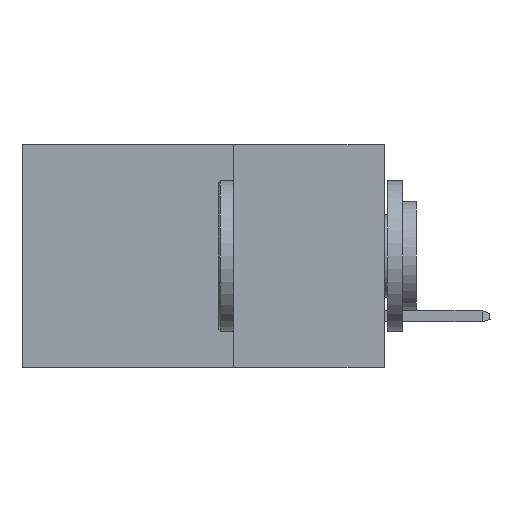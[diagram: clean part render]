
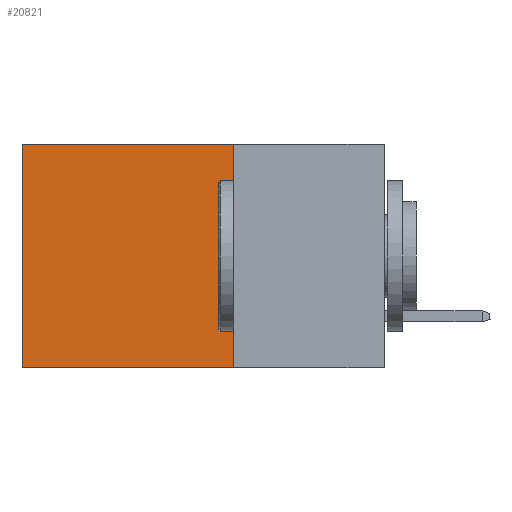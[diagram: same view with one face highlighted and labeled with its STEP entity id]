
A CAD part, left-side view. The second image highlights one B-rep face of the part: STEP entity #20821.
In plain terms, the highlighted planar face has unit normal (-1, 0, 0).
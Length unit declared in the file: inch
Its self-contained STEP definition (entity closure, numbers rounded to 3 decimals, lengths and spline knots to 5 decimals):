
#417 = VECTOR ( 'NONE', #20876, 39.37008 ) ;
#2140 = ORIENTED_EDGE ( 'NONE', *, *, #23260, .T. ) ;
#3273 = CARTESIAN_POINT ( 'NONE',  ( 0.298, 0.25, -0.37 ) ) ;
#4256 = EDGE_LOOP ( 'NONE', ( #18175, #8787, #15003, #2140 ) ) ;
#5755 = VERTEX_POINT ( 'NONE', #19943 ) ;
#6145 = CARTESIAN_POINT ( 'NONE',  ( 0.298, 0.25, 0. ) ) ;
#6293 = DIRECTION ( 'NONE',  ( 0., 0., -1. ) ) ;
#7653 = EDGE_CURVE ( 'NONE', #23555, #8686, #29731, .T. ) ;
#8686 = VERTEX_POINT ( 'NONE', #3273 ) ;
#8787 = ORIENTED_EDGE ( 'NONE', *, *, #19134, .F. ) ;
#10537 = CARTESIAN_POINT ( 'NONE',  ( 0.298, 0.25, 0. ) ) ;
#11476 = DIRECTION ( 'NONE',  ( 0., 0., -1. ) ) ;
#13625 = LINE ( 'NONE', #18662, #417 ) ;
#13712 = VECTOR ( 'NONE', #26674, 39.37008 ) ;
#15003 = ORIENTED_EDGE ( 'NONE', *, *, #7653, .F. ) ;
#15560 = EDGE_CURVE ( 'NONE', #5755, #27380, #30131, .T. ) ;
#17323 = DIRECTION ( 'NONE',  ( 0., 0., -1. ) ) ;
#18148 = CARTESIAN_POINT ( 'NONE',  ( 0.298, 0.25, 0. ) ) ;
#18175 = ORIENTED_EDGE ( 'NONE', *, *, #15560, .T. ) ;
#18662 = CARTESIAN_POINT ( 'NONE',  ( 0.298, 0.25, -0.37 ) ) ;
#19134 = EDGE_CURVE ( 'NONE', #8686, #27380, #13625, .T. ) ;
#19943 = CARTESIAN_POINT ( 'NONE',  ( 0.298, 0.6, 0. ) ) ;
#20821 = ADVANCED_FACE ( 'NONE', ( #21860 ), #29582, .F. ) ;
#20876 = DIRECTION ( 'NONE',  ( 0., 1., 0. ) ) ;
#21416 = CARTESIAN_POINT ( 'NONE',  ( 0.298, 0.6, 0. ) ) ;
#21860 = FACE_OUTER_BOUND ( 'NONE', #4256, .T. ) ;
#22546 = VECTOR ( 'NONE', #6293, 39.37008 ) ;
#23260 = EDGE_CURVE ( 'NONE', #23555, #5755, #26596, .T. ) ;
#23555 = VERTEX_POINT ( 'NONE', #6145 ) ;
#24356 = CARTESIAN_POINT ( 'NONE',  ( 0.298, 0.25, 0. ) ) ;
#24907 = DIRECTION ( 'NONE',  ( 1., 0., 0. ) ) ;
#26332 = VECTOR ( 'NONE', #11476, 39.37008 ) ;
#26596 = LINE ( 'NONE', #24356, #13712 ) ;
#26674 = DIRECTION ( 'NONE',  ( 0., 1., 0. ) ) ;
#27150 = CARTESIAN_POINT ( 'NONE',  ( 0.298, 0.6, -0.37 ) ) ;
#27380 = VERTEX_POINT ( 'NONE', #27150 ) ;
#27572 = AXIS2_PLACEMENT_3D ( 'NONE', #10537, #24907, #17323 ) ;
#29582 = PLANE ( 'NONE',  #27572 ) ;
#29731 = LINE ( 'NONE', #18148, #22546 ) ;
#30131 = LINE ( 'NONE', #21416, #26332 ) ;
